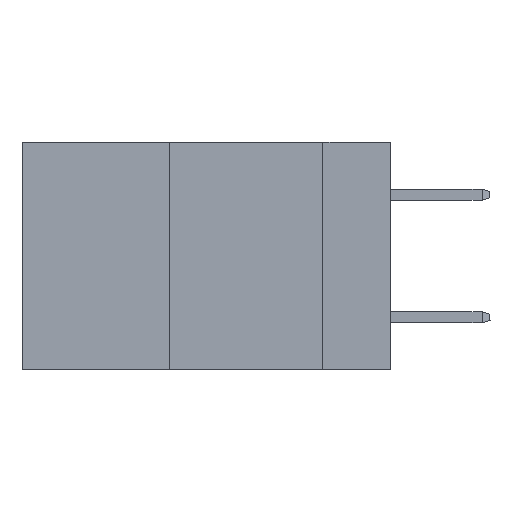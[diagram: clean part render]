
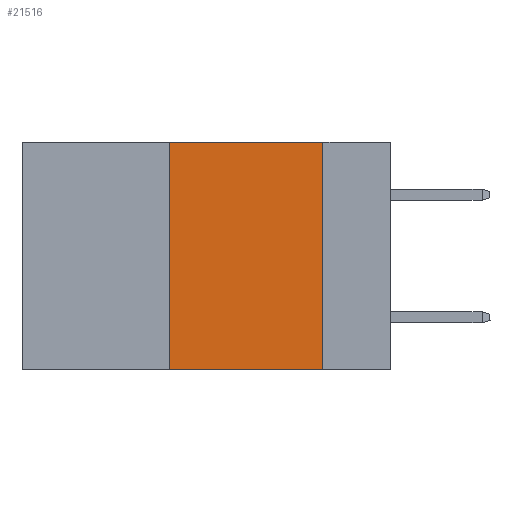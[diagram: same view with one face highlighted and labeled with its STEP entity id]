
A CAD part, left-side view. The second image highlights one B-rep face of the part: STEP entity #21516.
In plain terms, the highlighted planar face has unit normal (-1, 0, 0).
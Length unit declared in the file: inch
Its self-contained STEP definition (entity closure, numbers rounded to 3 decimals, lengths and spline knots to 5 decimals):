
#640 = LINE ( 'NONE', #14497, #12014 ) ;
#1300 = ORIENTED_EDGE ( 'NONE', *, *, #28322, .F. ) ;
#1440 = CARTESIAN_POINT ( 'NONE',  ( 0., 0.11, 0. ) ) ;
#3149 = PLANE ( 'NONE',  #23424 ) ;
#4806 = VERTEX_POINT ( 'NONE', #36893 ) ;
#4987 = ORIENTED_EDGE ( 'NONE', *, *, #38610, .F. ) ;
#5173 = LINE ( 'NONE', #42831, #39443 ) ;
#5981 = CARTESIAN_POINT ( 'NONE',  ( 0., 0.11, -0.37 ) ) ;
#6462 = CARTESIAN_POINT ( 'NONE',  ( 0., 0.6, 0. ) ) ;
#7124 = VERTEX_POINT ( 'NONE', #42163 ) ;
#7896 = EDGE_CURVE ( 'NONE', #7124, #4806, #5173, .T. ) ;
#9779 = DIRECTION ( 'NONE',  ( 0., 0., -1. ) ) ;
#10441 = DIRECTION ( 'NONE',  ( 0., 0., 1. ) ) ;
#10580 = CARTESIAN_POINT ( 'NONE',  ( 0., 0.36, 0. ) ) ;
#12014 = VECTOR ( 'NONE', #37440, 39.37008 ) ;
#12304 = VECTOR ( 'NONE', #10441, 39.37008 ) ;
#14497 = CARTESIAN_POINT ( 'NONE',  ( 0., 0.6, -0.37 ) ) ;
#14805 = FACE_OUTER_BOUND ( 'NONE', #16517, .T. ) ;
#14883 = VERTEX_POINT ( 'NONE', #5981 ) ;
#16517 = EDGE_LOOP ( 'NONE', ( #1300, #38831, #4987, #17597 ) ) ;
#17597 = ORIENTED_EDGE ( 'NONE', *, *, #31645, .T. ) ;
#19503 = DIRECTION ( 'NONE',  ( 0., -1., 0. ) ) ;
#21516 = ADVANCED_FACE ( 'NONE', ( #14805 ), #3149, .F. ) ;
#21773 = VERTEX_POINT ( 'NONE', #42042 ) ;
#23424 = AXIS2_PLACEMENT_3D ( 'NONE', #6462, #29735, #9779 ) ;
#26679 = LINE ( 'NONE', #1440, #32892 ) ;
#26972 = LINE ( 'NONE', #10580, #12304 ) ;
#28322 = EDGE_CURVE ( 'NONE', #4806, #14883, #26679, .T. ) ;
#29735 = DIRECTION ( 'NONE',  ( 1., 0., 0. ) ) ;
#31645 = EDGE_CURVE ( 'NONE', #21773, #14883, #640, .T. ) ;
#32892 = VECTOR ( 'NONE', #38789, 39.37008 ) ;
#36893 = CARTESIAN_POINT ( 'NONE',  ( 0., 0.11, 0. ) ) ;
#37440 = DIRECTION ( 'NONE',  ( 0., -1., 0. ) ) ;
#38610 = EDGE_CURVE ( 'NONE', #21773, #7124, #26972, .T. ) ;
#38789 = DIRECTION ( 'NONE',  ( 0., 0., -1. ) ) ;
#38831 = ORIENTED_EDGE ( 'NONE', *, *, #7896, .F. ) ;
#39443 = VECTOR ( 'NONE', #19503, 39.37008 ) ;
#42042 = CARTESIAN_POINT ( 'NONE',  ( 0., 0.36, -0.37 ) ) ;
#42163 = CARTESIAN_POINT ( 'NONE',  ( 0., 0.36, 0. ) ) ;
#42831 = CARTESIAN_POINT ( 'NONE',  ( 0., 0.6, 0. ) ) ;
